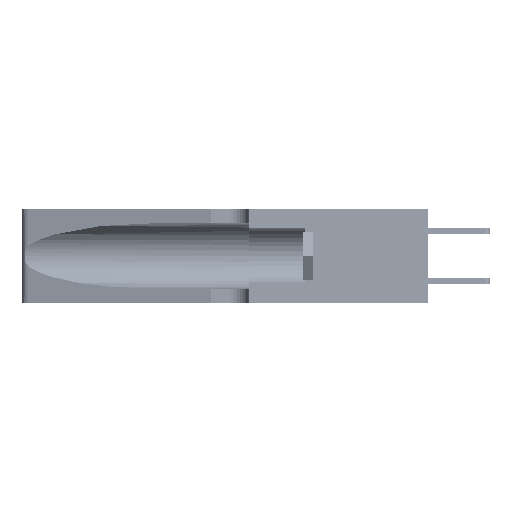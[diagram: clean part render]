
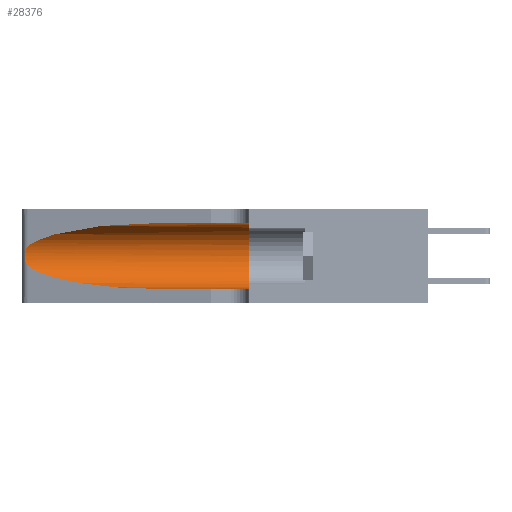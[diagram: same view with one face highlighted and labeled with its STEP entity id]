
A CAD part, left-side view. The second image highlights one B-rep face of the part: STEP entity #28376.
In plain terms, the highlighted cylindrical face has radius 3.308 mm (diameter 6.617 mm), a partial arc.
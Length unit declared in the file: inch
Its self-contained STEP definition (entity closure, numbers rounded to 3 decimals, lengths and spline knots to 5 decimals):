
#394 = VERTEX_POINT ( 'NONE', #45255 ) ;
#756 = CARTESIAN_POINT ( 'NONE',  ( 0.25555, 1.22994, 0.2215 ) ) ;
#1093 = CARTESIAN_POINT ( 'NONE',  ( 0.26017, 1.23833, 0.17102 ) ) ;
#2582 = EDGE_LOOP ( 'NONE', ( #16770, #49330, #30390, #44553, #47992, #28568 ) ) ;
#4657 = EDGE_CURVE ( 'NONE', #26090, #19690, #40550, .T. ) ;
#5052 = CARTESIAN_POINT ( 'NONE',  ( 0.25487, 1.22718, 0.14631 ) ) ;
#5367 = CARTESIAN_POINT ( 'NONE',  ( 0.18966, 0.96281, 0.31525 ) ) ;
#5832 = CARTESIAN_POINT ( 'NONE',  ( 0.25789, 1.23486, 0.15765 ) ) ;
#9307 = CARTESIAN_POINT ( 'NONE',  ( 0.1305, 0.72297, 0.05475 ) ) ;
#14642 = DIRECTION ( 'NONE',  ( 0., 1., 0. ) ) ;
#16428 = CARTESIAN_POINT ( 'NONE',  ( 0.25787, 1.23484, 0.2124 ) ) ;
#16741 = CYLINDRICAL_SURFACE ( 'NONE', #21577, 0.13025 ) ;
#16770 = ORIENTED_EDGE ( 'NONE', *, *, #44500, .T. ) ;
#16781 = CARTESIAN_POINT ( 'NONE',  ( 0.25487, 1.22718, 0.22369 ) ) ;
#17125 = CARTESIAN_POINT ( 'NONE',  ( 0.25639, 1.23186, 0.15144 ) ) ;
#17308 = CARTESIAN_POINT ( 'NONE',  ( 0.26075, 1.23896, 0.178 ) ) ;
#19156 = VECTOR ( 'NONE', #35717, 39.37008 ) ;
#19690 = VERTEX_POINT ( 'NONE', #43178 ) ;
#19796 = CARTESIAN_POINT ( 'NONE',  ( 0.25487, 1.22718, 0.14631 ) ) ;
#21577 = AXIS2_PLACEMENT_3D ( 'NONE', #37168, #40728, #48813 ) ;
#21753 = CIRCLE ( 'NONE', #37728, 0.13025 ) ;
#23263 = CARTESIAN_POINT ( 'NONE',  ( 0.1305, 1.61858, 0.05475 ) ) ;
#24141 = DIRECTION ( 'NONE',  ( 0., -1., 0. ) ) ;
#24528 = CARTESIAN_POINT ( 'NONE',  ( 0.25639, 1.23184, 0.21858 ) ) ;
#25224 = CARTESIAN_POINT ( 'NONE',  ( 0.25487, 1.22718, 0.14631 ) ) ;
#25495 = EDGE_CURVE ( 'NONE', #36637, #33092, #39684, .T. ) ;
#25792 = EDGE_CURVE ( 'NONE', #394, #33099, #39664, .T. ) ;
#26090 = VERTEX_POINT ( 'NONE', #9307 ) ;
#28376 = ADVANCED_FACE ( 'NONE', ( #46323 ), #16741, .F. ) ;
#28568 = ORIENTED_EDGE ( 'NONE', *, *, #25792, .F. ) ;
#28607 = EDGE_CURVE ( 'NONE', #33099, #19690, #21753, .T. ) ;
#29431 = CARTESIAN_POINT ( 'NONE',  ( 0.25856, 1.23593, 0.16098 ) ) ;
#30390 = ORIENTED_EDGE ( 'NONE', *, *, #34076, .T. ) ;
#31325 = CARTESIAN_POINT ( 'NONE',  ( 0.1305, 1.61858, 0.31525 ) ) ;
#33092 = VERTEX_POINT ( 'NONE', #5052 ) ;
#33099 = VERTEX_POINT ( 'NONE', #45345 ) ;
#33472 = CARTESIAN_POINT ( 'NONE',  ( 0.25555, 1.22993, 0.14849 ) ) ;
#33522 = CARTESIAN_POINT ( 'NONE',  ( 0.1305, 0.72297, 0.31525 ) ) ;
#34076 = EDGE_CURVE ( 'NONE', #33092, #26090, #49975, .T. ) ;
#35420 = CARTESIAN_POINT ( 'NONE',  ( 0.18966, 0.96281, 0.05475 ) ) ;
#35717 = DIRECTION ( 'NONE',  ( 0., -1., 0. ) ) ;
#35850 = VECTOR ( 'NONE', #24141, 39.37008 ) ;
#36637 = VERTEX_POINT ( 'NONE', #39261 ) ;
#37168 = CARTESIAN_POINT ( 'NONE',  ( 0.1305, 1.61858, 0.185 ) ) ;
#37391 = CARTESIAN_POINT ( 'NONE',  ( 0.2373, 1.15595, 0.28018 ) ) ;
#37728 = AXIS2_PLACEMENT_3D ( 'NONE', #46493, #14642, #50529 ) ;
#39261 = CARTESIAN_POINT ( 'NONE',  ( 0.25487, 1.22718, 0.22369 ) ) ;
#39664 = LINE ( 'NONE', #31325, #35850 ) ;
#39684 = B_SPLINE_CURVE_WITH_KNOTS ( 'NONE', 3,
 ( #16781, #756, #24528, #16428, #44589, #45443, #41232, #17308, #1093, #29431, #5832, #17125, #33472, #25224 ),
 .UNSPECIFIED., .F., .F.,
 ( 4, 2, 2, 2, 2, 2, 4 ),
 ( 0., 0.00027, 0.00053, 0.00107, 0.0016, 0.00187, 0.00214 ),
 .UNSPECIFIED. ) ;
#40550 = LINE ( 'NONE', #23263, #19156 ) ;
#40728 = DIRECTION ( 'NONE',  ( 0., -1., 0. ) ) ;
#41232 = CARTESIAN_POINT ( 'NONE',  ( 0.26075, 1.23896, 0.19203 ) ) ;
#41608 = CARTESIAN_POINT ( 'NONE',  ( 0.25487, 1.22718, 0.22369 ) ) ;
#43178 = CARTESIAN_POINT ( 'NONE',  ( 0.1305, 0.35, 0.05475 ) ) ;
#43542 = CARTESIAN_POINT ( 'NONE',  ( 0.2373, 1.15595, 0.08982 ) ) ;
#43853 =( BOUNDED_CURVE ( )  B_SPLINE_CURVE ( 3, ( #33522, #5367, #37391, #41608 ),
 .UNSPECIFIED., .F., .F. ) 
 B_SPLINE_CURVE_WITH_KNOTS ( ( 4, 4 ),
 ( 1.5708, 2.84003 ),
 .UNSPECIFIED. ) 
 CURVE ( )  GEOMETRIC_REPRESENTATION_ITEM ( )  RATIONAL_B_SPLINE_CURVE ( ( 1., 0.87, 0.87, 1. ) ) 
 REPRESENTATION_ITEM ( '' )  );
#44500 = EDGE_CURVE ( 'NONE', #394, #36637, #43853, .T. ) ;
#44553 = ORIENTED_EDGE ( 'NONE', *, *, #4657, .T. ) ;
#44589 = CARTESIAN_POINT ( 'NONE',  ( 0.25854, 1.2359, 0.20912 ) ) ;
#45255 = CARTESIAN_POINT ( 'NONE',  ( 0.1305, 0.72297, 0.31525 ) ) ;
#45345 = CARTESIAN_POINT ( 'NONE',  ( 0.1305, 0.35, 0.31525 ) ) ;
#45443 = CARTESIAN_POINT ( 'NONE',  ( 0.26018, 1.23835, 0.19895 ) ) ;
#46323 = FACE_OUTER_BOUND ( 'NONE', #2582, .T. ) ;
#46493 = CARTESIAN_POINT ( 'NONE',  ( 0.1305, 0.35, 0.185 ) ) ;
#47992 = ORIENTED_EDGE ( 'NONE', *, *, #28607, .F. ) ;
#48813 = DIRECTION ( 'NONE',  ( 0., 0., -1. ) ) ;
#49330 = ORIENTED_EDGE ( 'NONE', *, *, #25495, .T. ) ;
#49975 =( BOUNDED_CURVE ( )  B_SPLINE_CURVE ( 3, ( #19796, #43542, #35420, #51597 ),
 .UNSPECIFIED., .F., .F. ) 
 B_SPLINE_CURVE_WITH_KNOTS ( ( 4, 4 ),
 ( 3.44316, 4.71239 ),
 .UNSPECIFIED. ) 
 CURVE ( )  GEOMETRIC_REPRESENTATION_ITEM ( )  RATIONAL_B_SPLINE_CURVE ( ( 1., 0.87, 0.87, 1. ) ) 
 REPRESENTATION_ITEM ( '' )  );
#50529 = DIRECTION ( 'NONE',  ( 0., 0., 1. ) ) ;
#51597 = CARTESIAN_POINT ( 'NONE',  ( 0.1305, 0.72297, 0.05475 ) ) ;
